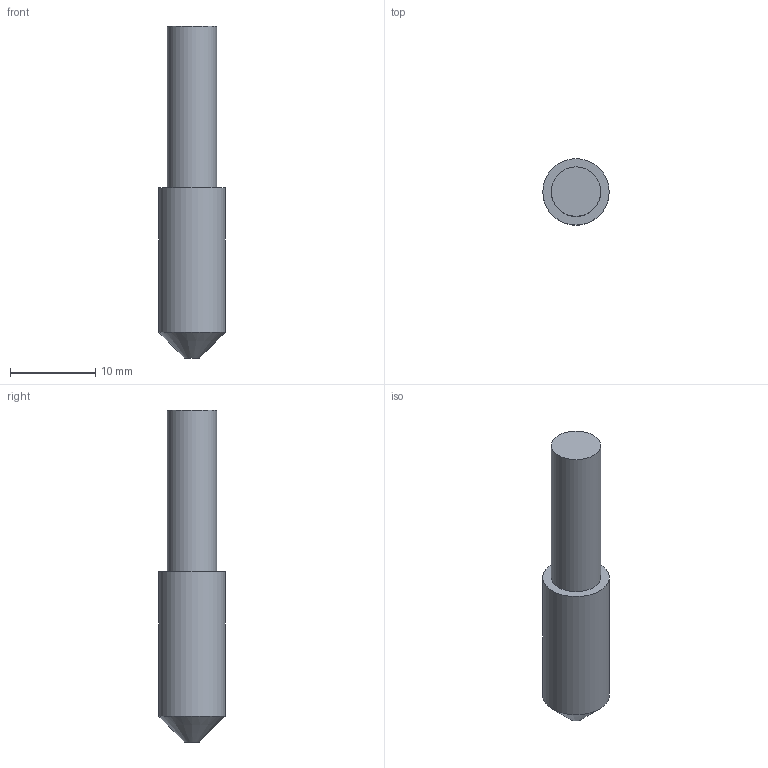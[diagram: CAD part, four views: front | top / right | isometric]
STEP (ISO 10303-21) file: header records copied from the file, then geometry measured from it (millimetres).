
FILE_DESCRIPTION (( 'STEP AP203' ), '1' );
FILE_NAME ('WTF-9_hillbilly_mag_catch_rod.STEP', '2020-05-09T08:59:46', ( '' ), ( '' ), 'SwSTEP 2.0', 'SolidWorks 2016', '' );
FILE_SCHEMA (( 'CONFIG_CONTROL_DESIGN' ));
Length unit declared in the file: millimetre
Products named in the file (2): WTF-9_hillbilly_mag_catch_rod; WTF HILLBILLY FINAL
Assembly tree (1 placements, depth 2):
  WTF-9_hillbilly_mag_catch_rod
    WTF HILLBILLY FINAL
Bounding box: 7.8 x 7.8 x 39 mm (x, y, z)
Volume: 1375.7 mm3; surface area: 877.1 mm2
Topology: 1 solids, 1 shells, 6 faces, 9 edges, 6 vertices
Faces by surface type: plane 3, cylinder 2, cone 1
Full cylindrical faces by diameter (mm): 5.8 x1, 7.8 x1
Entity records: 310 total; most frequent: DIRECTION 30, CARTESIAN_POINT 20, PERSON_AND_ORGANIZATION 17, AXIS2_PLACEMENT_3D 15, CALENDAR_DATE 12, COORDINATED_UNIVERSAL_TIME_OFFSET 12, LOCAL_TIME 12, DATE_AND_TIME 12
